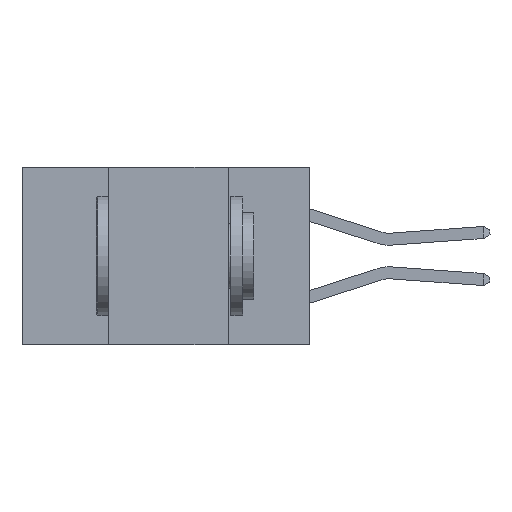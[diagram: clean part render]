
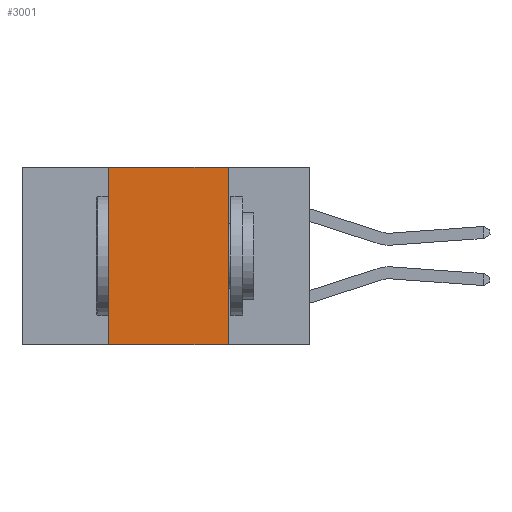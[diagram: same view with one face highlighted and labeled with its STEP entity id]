
A CAD part, left-side view. The second image highlights one B-rep face of the part: STEP entity #3001.
In plain terms, the highlighted planar face has unit normal (-1, 0, 0).
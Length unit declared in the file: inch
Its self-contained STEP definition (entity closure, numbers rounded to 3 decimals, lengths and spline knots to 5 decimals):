
#7 = FACE_OUTER_BOUND ( 'NONE', #7109, .T. ) ;
#25 = VERTEX_POINT ( 'NONE', #5295 ) ;
#1435 = AXIS2_PLACEMENT_3D ( 'NONE', #14801, #13065, #12860 ) ;
#1587 = VERTEX_POINT ( 'NONE', #5470 ) ;
#2119 = VERTEX_POINT ( 'NONE', #5816 ) ;
#2231 = VECTOR ( 'NONE', #6525, 39.37008 ) ;
#2659 = VERTEX_POINT ( 'NONE', #10004 ) ;
#3001 = ADVANCED_FACE ( 'NONE', ( #7 ), #14811, .F. ) ;
#3464 = CARTESIAN_POINT ( 'NONE',  ( 0., 0.6, -0.37 ) ) ;
#3513 = DIRECTION ( 'NONE',  ( 0., -1., 0. ) ) ;
#3779 = ORIENTED_EDGE ( 'NONE', *, *, #10514, .F. ) ;
#4254 = LINE ( 'NONE', #3464, #7315 ) ;
#4837 = ORIENTED_EDGE ( 'NONE', *, *, #10845, .T. ) ;
#5295 = CARTESIAN_POINT ( 'NONE',  ( 0., 0.17, 0. ) ) ;
#5470 = CARTESIAN_POINT ( 'NONE',  ( 0., 0.42, -0.37 ) ) ;
#5816 = CARTESIAN_POINT ( 'NONE',  ( 0., 0.17, -0.37 ) ) ;
#6525 = DIRECTION ( 'NONE',  ( 0., 0., 1. ) ) ;
#6560 = CARTESIAN_POINT ( 'NONE',  ( 0., 0.42, 0. ) ) ;
#7109 = EDGE_LOOP ( 'NONE', ( #13473, #12566, #3779, #4837 ) ) ;
#7315 = VECTOR ( 'NONE', #3513, 39.37008 ) ;
#8356 = DIRECTION ( 'NONE',  ( 0., -1., 0. ) ) ;
#8476 = EDGE_CURVE ( 'NONE', #25, #2119, #14397, .T. ) ;
#8602 = VECTOR ( 'NONE', #8356, 39.37008 ) ;
#8962 = LINE ( 'NONE', #10674, #8602 ) ;
#10004 = CARTESIAN_POINT ( 'NONE',  ( 0., 0.42, 0. ) ) ;
#10514 = EDGE_CURVE ( 'NONE', #1587, #2659, #14691, .T. ) ;
#10674 = CARTESIAN_POINT ( 'NONE',  ( 0., 0.6, 0. ) ) ;
#10845 = EDGE_CURVE ( 'NONE', #1587, #2119, #4254, .T. ) ;
#12566 = ORIENTED_EDGE ( 'NONE', *, *, #13810, .F. ) ;
#12860 = DIRECTION ( 'NONE',  ( 0., 0., -1. ) ) ;
#12863 = DIRECTION ( 'NONE',  ( 0., 0., -1. ) ) ;
#13065 = DIRECTION ( 'NONE',  ( 1., 0., 0. ) ) ;
#13473 = ORIENTED_EDGE ( 'NONE', *, *, #8476, .F. ) ;
#13693 = VECTOR ( 'NONE', #12863, 39.37008 ) ;
#13810 = EDGE_CURVE ( 'NONE', #2659, #25, #8962, .T. ) ;
#14335 = CARTESIAN_POINT ( 'NONE',  ( 0., 0.17, 0. ) ) ;
#14397 = LINE ( 'NONE', #14335, #13693 ) ;
#14691 = LINE ( 'NONE', #6560, #2231 ) ;
#14801 = CARTESIAN_POINT ( 'NONE',  ( 0., 0.6, 0. ) ) ;
#14811 = PLANE ( 'NONE',  #1435 ) ;
